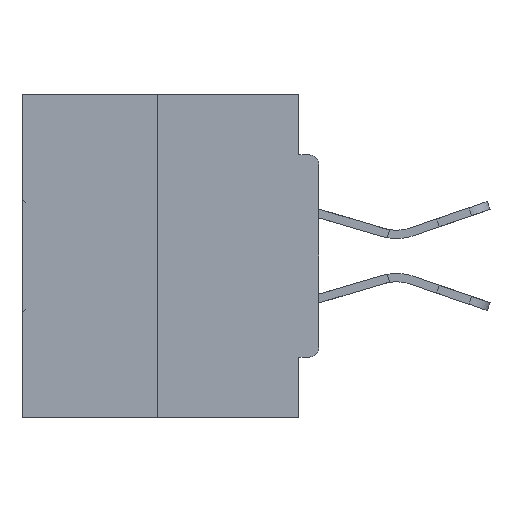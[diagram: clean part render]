
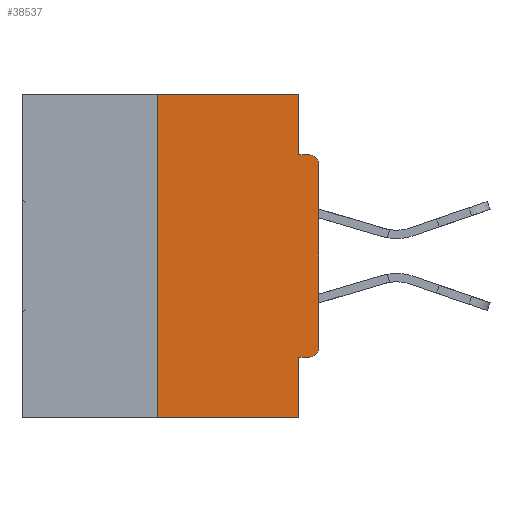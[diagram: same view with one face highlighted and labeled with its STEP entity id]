
A CAD part, left-side view. The second image highlights one B-rep face of the part: STEP entity #38537.
In plain terms, the highlighted planar face has unit normal (-1, 0, 0).
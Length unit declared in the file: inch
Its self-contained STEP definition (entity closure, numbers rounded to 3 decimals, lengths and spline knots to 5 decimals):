
#320 = FACE_OUTER_BOUND ( 'NONE', #15919, .T. ) ;
#497 = ORIENTED_EDGE ( 'NONE', *, *, #36564, .F. ) ;
#560 = LINE ( 'NONE', #29017, #29028 ) ;
#1661 = LINE ( 'NONE', #10932, #25660 ) ;
#1664 = ORIENTED_EDGE ( 'NONE', *, *, #13720, .T. ) ;
#2147 = VERTEX_POINT ( 'NONE', #5946 ) ;
#2434 = EDGE_CURVE ( 'NONE', #7428, #10010, #24047, .T. ) ;
#3237 = VECTOR ( 'NONE', #14959, 39.37008 ) ;
#4319 = CARTESIAN_POINT ( 'NONE',  ( 0., 0., -0.1085 ) ) ;
#4384 = DIRECTION ( 'NONE',  ( 0., 0., -1. ) ) ;
#4838 = VECTOR ( 'NONE', #8026, 39.37008 ) ;
#5946 = CARTESIAN_POINT ( 'NONE',  ( 0., 0.015, -0.0935 ) ) ;
#6027 = LINE ( 'NONE', #44068, #3237 ) ;
#6052 = VERTEX_POINT ( 'NONE', #23387 ) ;
#6169 = PLANE ( 'NONE',  #15144 ) ;
#6394 = ORIENTED_EDGE ( 'NONE', *, *, #2434, .T. ) ;
#6704 = CARTESIAN_POINT ( 'NONE',  ( 0., 0.031, 0. ) ) ;
#6766 = AXIS2_PLACEMENT_3D ( 'NONE', #25727, #36376, #26062 ) ;
#7085 = ORIENTED_EDGE ( 'NONE', *, *, #45564, .F. ) ;
#7408 = EDGE_CURVE ( 'NONE', #43390, #6052, #17386, .T. ) ;
#7428 = VERTEX_POINT ( 'NONE', #40465 ) ;
#8026 = DIRECTION ( 'NONE',  ( 0., 0., 1. ) ) ;
#8391 = VERTEX_POINT ( 'NONE', #4319 ) ;
#10010 = VERTEX_POINT ( 'NONE', #41359 ) ;
#10932 = CARTESIAN_POINT ( 'NONE',  ( 0., 0.031, 0. ) ) ;
#11717 = VERTEX_POINT ( 'NONE', #6704 ) ;
#12953 = VERTEX_POINT ( 'NONE', #25232 ) ;
#13122 = CIRCLE ( 'NONE', #35795, 0.015 ) ;
#13720 = EDGE_CURVE ( 'NONE', #6052, #8391, #6027, .T. ) ;
#14940 = CARTESIAN_POINT ( 'NONE',  ( 0., 0., -0.4065 ) ) ;
#14959 = DIRECTION ( 'NONE',  ( 0., 0., 1. ) ) ;
#15144 = AXIS2_PLACEMENT_3D ( 'NONE', #41719, #24119, #23804 ) ;
#15919 = EDGE_LOOP ( 'NONE', ( #7085, #38302, #6394, #497, #39624, #44475, #1664, #22386, #20383, #38600 ) ) ;
#16711 = CARTESIAN_POINT ( 'NONE',  ( 0., 0.015, -0.4065 ) ) ;
#17234 = DIRECTION ( 'NONE',  ( 0., 0., -1. ) ) ;
#17386 = CIRCLE ( 'NONE', #6766, 0.015 ) ;
#17480 = CARTESIAN_POINT ( 'NONE',  ( 0., 0.46, -0.5 ) ) ;
#17996 = EDGE_CURVE ( 'NONE', #43390, #43098, #24215, .T. ) ;
#18063 = DIRECTION ( 'NONE',  ( 0., 0., -1. ) ) ;
#18983 = DIRECTION ( 'NONE',  ( 0., -1., 0. ) ) ;
#19192 = VECTOR ( 'NONE', #39822, 39.37008 ) ;
#19343 = LINE ( 'NONE', #40697, #4838 ) ;
#20383 = ORIENTED_EDGE ( 'NONE', *, *, #41201, .F. ) ;
#21656 = VECTOR ( 'NONE', #17234, 39.37008 ) ;
#22386 = ORIENTED_EDGE ( 'NONE', *, *, #27037, .T. ) ;
#22597 = EDGE_CURVE ( 'NONE', #7428, #12953, #19343, .T. ) ;
#23387 = CARTESIAN_POINT ( 'NONE',  ( 0., 0., -0.3915 ) ) ;
#23804 = DIRECTION ( 'NONE',  ( 0., 0., -1. ) ) ;
#24047 = LINE ( 'NONE', #17480, #42023 ) ;
#24119 = DIRECTION ( 'NONE',  ( 1., 0., 0. ) ) ;
#24215 = LINE ( 'NONE', #14940, #19192 ) ;
#25232 = CARTESIAN_POINT ( 'NONE',  ( 0., 0.25, 0. ) ) ;
#25660 = VECTOR ( 'NONE', #18063, 39.37008 ) ;
#25727 = CARTESIAN_POINT ( 'NONE',  ( 0., 0.015, -0.3915 ) ) ;
#26062 = DIRECTION ( 'NONE',  ( 0., 0., -1. ) ) ;
#27037 = EDGE_CURVE ( 'NONE', #8391, #2147, #13122, .T. ) ;
#27992 = LINE ( 'NONE', #36683, #38106 ) ;
#28708 = CARTESIAN_POINT ( 'NONE',  ( 0., 0.031, -0.4065 ) ) ;
#29017 = CARTESIAN_POINT ( 'NONE',  ( 0., 0.46, 0. ) ) ;
#29028 = VECTOR ( 'NONE', #29653, 39.37008 ) ;
#29653 = DIRECTION ( 'NONE',  ( 0., -1., 0. ) ) ;
#29883 = EDGE_CURVE ( 'NONE', #11717, #39864, #1661, .T. ) ;
#30476 = CARTESIAN_POINT ( 'NONE',  ( 0., 0.031, -0.0935 ) ) ;
#31313 = CARTESIAN_POINT ( 'NONE',  ( 0., 0.031, -0.5 ) ) ;
#32517 = DIRECTION ( 'NONE',  ( -1., 0., 0. ) ) ;
#35173 = DIRECTION ( 'NONE',  ( 0., -1., 0. ) ) ;
#35795 = AXIS2_PLACEMENT_3D ( 'NONE', #36128, #32517, #4384 ) ;
#36128 = CARTESIAN_POINT ( 'NONE',  ( 0., 0.015, -0.1085 ) ) ;
#36376 = DIRECTION ( 'NONE',  ( -1., 0., 0. ) ) ;
#36564 = EDGE_CURVE ( 'NONE', #43098, #10010, #45232, .T. ) ;
#36683 = CARTESIAN_POINT ( 'NONE',  ( 0., 0., -0.0935 ) ) ;
#38106 = VECTOR ( 'NONE', #18983, 39.37008 ) ;
#38302 = ORIENTED_EDGE ( 'NONE', *, *, #22597, .F. ) ;
#38537 = ADVANCED_FACE ( 'NONE', ( #320 ), #6169, .F. ) ;
#38600 = ORIENTED_EDGE ( 'NONE', *, *, #29883, .F. ) ;
#39624 = ORIENTED_EDGE ( 'NONE', *, *, #17996, .F. ) ;
#39822 = DIRECTION ( 'NONE',  ( 0., 1., 0. ) ) ;
#39864 = VERTEX_POINT ( 'NONE', #30476 ) ;
#40465 = CARTESIAN_POINT ( 'NONE',  ( 0., 0.25, -0.5 ) ) ;
#40697 = CARTESIAN_POINT ( 'NONE',  ( 0., 0.25, 0. ) ) ;
#41201 = EDGE_CURVE ( 'NONE', #39864, #2147, #27992, .T. ) ;
#41359 = CARTESIAN_POINT ( 'NONE',  ( 0., 0.031, -0.5 ) ) ;
#41719 = CARTESIAN_POINT ( 'NONE',  ( 0., 0.46, 0. ) ) ;
#42023 = VECTOR ( 'NONE', #35173, 39.37008 ) ;
#43098 = VERTEX_POINT ( 'NONE', #28708 ) ;
#43390 = VERTEX_POINT ( 'NONE', #16711 ) ;
#44068 = CARTESIAN_POINT ( 'NONE',  ( 0., 0., 0. ) ) ;
#44475 = ORIENTED_EDGE ( 'NONE', *, *, #7408, .T. ) ;
#45232 = LINE ( 'NONE', #31313, #21656 ) ;
#45564 = EDGE_CURVE ( 'NONE', #12953, #11717, #560, .T. ) ;
